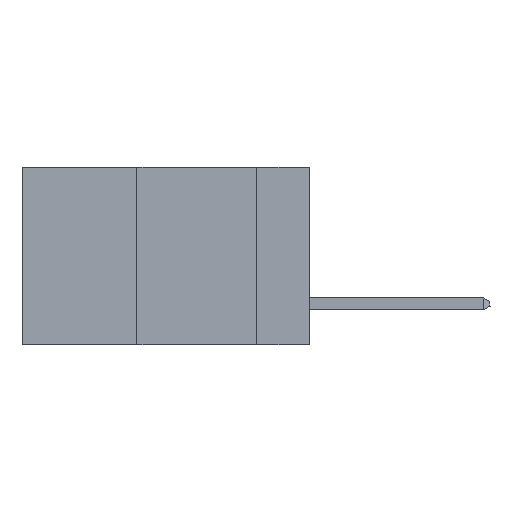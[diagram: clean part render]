
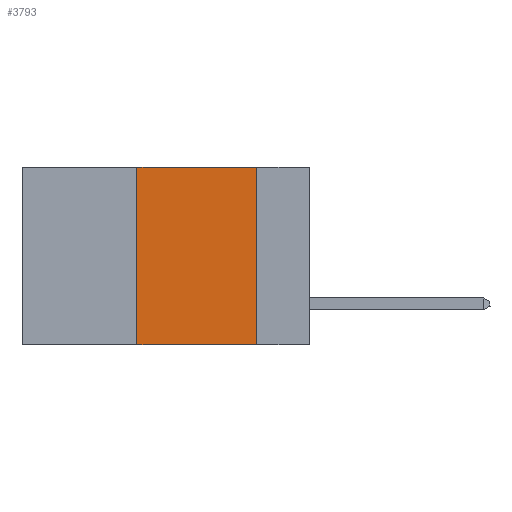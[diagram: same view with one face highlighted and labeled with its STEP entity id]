
A CAD part, left-side view. The second image highlights one B-rep face of the part: STEP entity #3793.
In plain terms, the highlighted planar face has unit normal (-1, 0, 0).
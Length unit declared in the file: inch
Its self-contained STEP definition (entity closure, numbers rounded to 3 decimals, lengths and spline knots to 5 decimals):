
#33 = CARTESIAN_POINT ( 'NONE',  ( 0., 0.6, 0. ) ) ;
#229 = EDGE_LOOP ( 'NONE', ( #2635, #9051, #6647, #1641 ) ) ;
#317 = CARTESIAN_POINT ( 'NONE',  ( 0., 0.36, 0. ) ) ;
#362 = DIRECTION ( 'NONE',  ( 0., 0., 1. ) ) ;
#384 = CARTESIAN_POINT ( 'NONE',  ( 0., 0.36, 0. ) ) ;
#1117 = EDGE_CURVE ( 'NONE', #1832, #1154, #7296, .T. ) ;
#1154 = VERTEX_POINT ( 'NONE', #2297 ) ;
#1641 = ORIENTED_EDGE ( 'NONE', *, *, #4146, .T. ) ;
#1702 = DIRECTION ( 'NONE',  ( 1., 0., 0. ) ) ;
#1832 = VERTEX_POINT ( 'NONE', #384 ) ;
#2297 = CARTESIAN_POINT ( 'NONE',  ( 0., 0.11, 0. ) ) ;
#2464 = EDGE_CURVE ( 'NONE', #8308, #1832, #3164, .T. ) ;
#2635 = ORIENTED_EDGE ( 'NONE', *, *, #6227, .F. ) ;
#2658 = VECTOR ( 'NONE', #4045, 39.37008 ) ;
#2663 = CARTESIAN_POINT ( 'NONE',  ( 0., 0.36, -0.37 ) ) ;
#3164 = LINE ( 'NONE', #317, #3303 ) ;
#3295 = CARTESIAN_POINT ( 'NONE',  ( 0., 0.6, -0.37 ) ) ;
#3303 = VECTOR ( 'NONE', #362, 39.37008 ) ;
#3394 = CARTESIAN_POINT ( 'NONE',  ( 0., 0.11, 0. ) ) ;
#3793 = ADVANCED_FACE ( 'NONE', ( #7638 ), #8161, .F. ) ;
#3867 = AXIS2_PLACEMENT_3D ( 'NONE', #9013, #1702, #4585 ) ;
#4045 = DIRECTION ( 'NONE',  ( 0., -1., 0. ) ) ;
#4146 = EDGE_CURVE ( 'NONE', #8308, #4284, #4184, .T. ) ;
#4184 = LINE ( 'NONE', #3295, #2658 ) ;
#4247 = LINE ( 'NONE', #3394, #6778 ) ;
#4284 = VERTEX_POINT ( 'NONE', #7148 ) ;
#4585 = DIRECTION ( 'NONE',  ( 0., 0., -1. ) ) ;
#4852 = VECTOR ( 'NONE', #9323, 39.37008 ) ;
#4905 = DIRECTION ( 'NONE',  ( 0., 0., -1. ) ) ;
#6227 = EDGE_CURVE ( 'NONE', #1154, #4284, #4247, .T. ) ;
#6647 = ORIENTED_EDGE ( 'NONE', *, *, #2464, .F. ) ;
#6778 = VECTOR ( 'NONE', #4905, 39.37008 ) ;
#7148 = CARTESIAN_POINT ( 'NONE',  ( 0., 0.11, -0.37 ) ) ;
#7296 = LINE ( 'NONE', #33, #4852 ) ;
#7638 = FACE_OUTER_BOUND ( 'NONE', #229, .T. ) ;
#8161 = PLANE ( 'NONE',  #3867 ) ;
#8308 = VERTEX_POINT ( 'NONE', #2663 ) ;
#9013 = CARTESIAN_POINT ( 'NONE',  ( 0., 0.6, 0. ) ) ;
#9051 = ORIENTED_EDGE ( 'NONE', *, *, #1117, .F. ) ;
#9323 = DIRECTION ( 'NONE',  ( 0., -1., 0. ) ) ;
